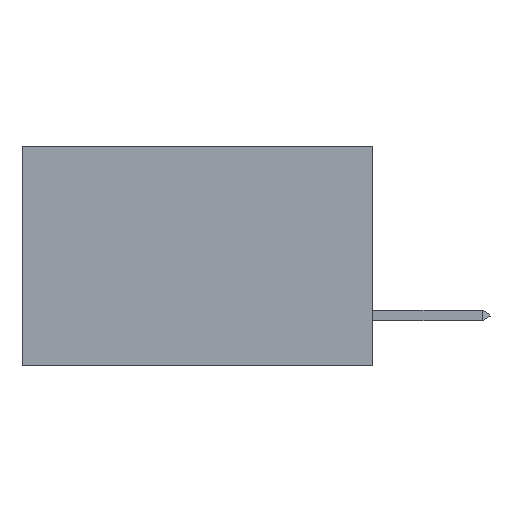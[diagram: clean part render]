
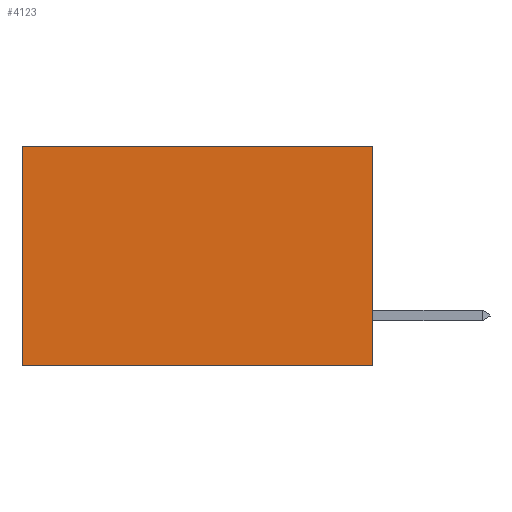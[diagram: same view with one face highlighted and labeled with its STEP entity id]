
A CAD part, left-side view. The second image highlights one B-rep face of the part: STEP entity #4123.
In plain terms, the highlighted planar face has unit normal (-1, 0, 0).
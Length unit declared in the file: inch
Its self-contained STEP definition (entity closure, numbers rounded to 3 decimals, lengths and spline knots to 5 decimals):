
#47 = CARTESIAN_POINT ( 'NONE',  ( 0.277, 0.59, 0. ) ) ;
#474 = DIRECTION ( 'NONE',  ( 0., 0., -1. ) ) ;
#765 = FACE_OUTER_BOUND ( 'NONE', #11506, .T. ) ;
#861 = ORIENTED_EDGE ( 'NONE', *, *, #11681, .F. ) ;
#1440 = DIRECTION ( 'NONE',  ( 0., 0., -1. ) ) ;
#1455 = DIRECTION ( 'NONE',  ( 1., 0., 0. ) ) ;
#1527 = CARTESIAN_POINT ( 'NONE',  ( 0.277, 0., -0.37 ) ) ;
#1551 = PLANE ( 'NONE',  #15376 ) ;
#2203 = EDGE_CURVE ( 'NONE', #17117, #4161, #14493, .T. ) ;
#2259 = CARTESIAN_POINT ( 'NONE',  ( 0.277, 0., -0.37 ) ) ;
#2642 = DIRECTION ( 'NONE',  ( 0., 1., 0. ) ) ;
#2980 = VECTOR ( 'NONE', #474, 39.37008 ) ;
#3381 = VECTOR ( 'NONE', #16267, 39.37008 ) ;
#4116 = LINE ( 'NONE', #9672, #8304 ) ;
#4123 = ADVANCED_FACE ( 'NONE', ( #765 ), #1551, .F. ) ;
#4161 = VERTEX_POINT ( 'NONE', #47 ) ;
#5603 = ORIENTED_EDGE ( 'NONE', *, *, #6486, .F. ) ;
#6486 = EDGE_CURVE ( 'NONE', #17117, #8283, #7182, .T. ) ;
#6696 = VECTOR ( 'NONE', #18142, 39.37008 ) ;
#7182 = LINE ( 'NONE', #17404, #2980 ) ;
#7770 = ORIENTED_EDGE ( 'NONE', *, *, #2203, .T. ) ;
#7911 = EDGE_CURVE ( 'NONE', #4161, #13352, #10420, .T. ) ;
#8283 = VERTEX_POINT ( 'NONE', #2259 ) ;
#8304 = VECTOR ( 'NONE', #2642, 39.37008 ) ;
#9672 = CARTESIAN_POINT ( 'NONE',  ( 0.277, 0., -0.37 ) ) ;
#10405 = CARTESIAN_POINT ( 'NONE',  ( 0.277, 0.59, -0.37 ) ) ;
#10420 = LINE ( 'NONE', #16767, #6696 ) ;
#11506 = EDGE_LOOP ( 'NONE', ( #17448, #861, #5603, #7770 ) ) ;
#11681 = EDGE_CURVE ( 'NONE', #8283, #13352, #4116, .T. ) ;
#13352 = VERTEX_POINT ( 'NONE', #10405 ) ;
#14278 = CARTESIAN_POINT ( 'NONE',  ( 0.277, 0., 0. ) ) ;
#14493 = LINE ( 'NONE', #17828, #3381 ) ;
#15376 = AXIS2_PLACEMENT_3D ( 'NONE', #1527, #1455, #1440 ) ;
#16267 = DIRECTION ( 'NONE',  ( 0., 1., 0. ) ) ;
#16767 = CARTESIAN_POINT ( 'NONE',  ( 0.277, 0.59, -0.37 ) ) ;
#17117 = VERTEX_POINT ( 'NONE', #14278 ) ;
#17404 = CARTESIAN_POINT ( 'NONE',  ( 0.277, 0., -0.37 ) ) ;
#17448 = ORIENTED_EDGE ( 'NONE', *, *, #7911, .T. ) ;
#17828 = CARTESIAN_POINT ( 'NONE',  ( 0.277, 0., 0. ) ) ;
#18142 = DIRECTION ( 'NONE',  ( 0., 0., -1. ) ) ;
